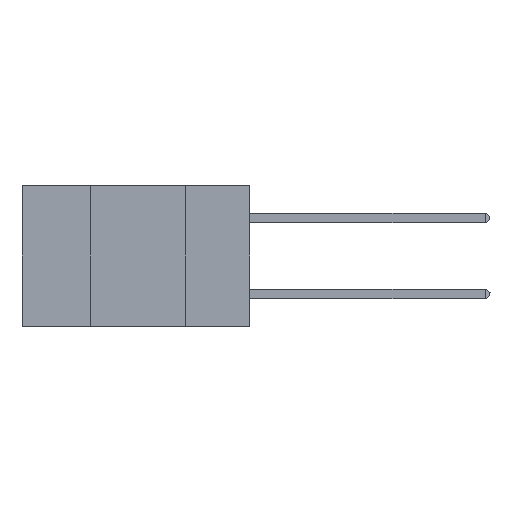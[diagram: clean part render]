
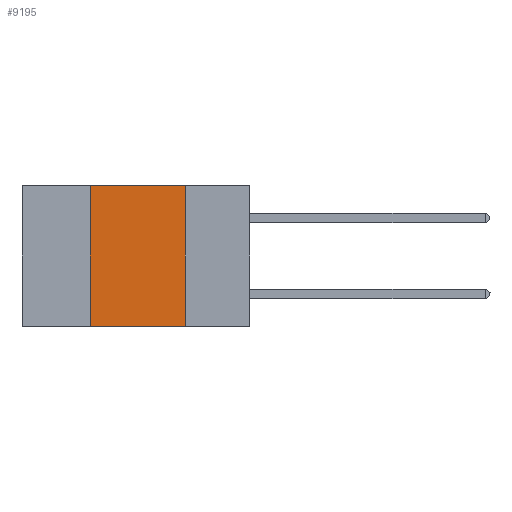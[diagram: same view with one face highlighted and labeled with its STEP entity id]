
A CAD part, left-side view. The second image highlights one B-rep face of the part: STEP entity #9195.
In plain terms, the highlighted planar face has unit normal (-1, 0, 0).
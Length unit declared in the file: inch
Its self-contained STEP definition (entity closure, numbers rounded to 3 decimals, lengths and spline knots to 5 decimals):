
#936 = CARTESIAN_POINT ( 'NONE',  ( 0., 0.6, -0.37 ) ) ;
#1093 = LINE ( 'NONE', #936, #21614 ) ;
#1607 = DIRECTION ( 'NONE',  ( 0., -1., 0. ) ) ;
#2502 = LINE ( 'NONE', #6776, #12777 ) ;
#3246 = CARTESIAN_POINT ( 'NONE',  ( 0., 0.42, 0. ) ) ;
#4138 = VECTOR ( 'NONE', #28139, 39.37008 ) ;
#4332 = ORIENTED_EDGE ( 'NONE', *, *, #9569, .T. ) ;
#4710 = DIRECTION ( 'NONE',  ( 0., 0., -1. ) ) ;
#5427 = DIRECTION ( 'NONE',  ( 0., 0., -1. ) ) ;
#5874 = CARTESIAN_POINT ( 'NONE',  ( 0., 0.42, -0.37 ) ) ;
#6187 = CARTESIAN_POINT ( 'NONE',  ( 0., 0.6, 0. ) ) ;
#6487 = CARTESIAN_POINT ( 'NONE',  ( 0., 0.6, 0. ) ) ;
#6776 = CARTESIAN_POINT ( 'NONE',  ( 0., 0.17, 0. ) ) ;
#7174 = VERTEX_POINT ( 'NONE', #7613 ) ;
#7613 = CARTESIAN_POINT ( 'NONE',  ( 0., 0.42, 0. ) ) ;
#7790 = PLANE ( 'NONE',  #30099 ) ;
#8316 = VERTEX_POINT ( 'NONE', #13761 ) ;
#8860 = VERTEX_POINT ( 'NONE', #16221 ) ;
#9195 = ADVANCED_FACE ( 'NONE', ( #13388 ), #7790, .F. ) ;
#9569 = EDGE_CURVE ( 'NONE', #30423, #8860, #1093, .T. ) ;
#11562 = EDGE_CURVE ( 'NONE', #30423, #7174, #17833, .T. ) ;
#12315 = ORIENTED_EDGE ( 'NONE', *, *, #11562, .F. ) ;
#12777 = VECTOR ( 'NONE', #4710, 39.37008 ) ;
#13388 = FACE_OUTER_BOUND ( 'NONE', #24349, .T. ) ;
#13509 = EDGE_CURVE ( 'NONE', #7174, #8316, #27596, .T. ) ;
#13697 = DIRECTION ( 'NONE',  ( 1., 0., 0. ) ) ;
#13761 = CARTESIAN_POINT ( 'NONE',  ( 0., 0.17, 0. ) ) ;
#15606 = EDGE_CURVE ( 'NONE', #8316, #8860, #2502, .T. ) ;
#16221 = CARTESIAN_POINT ( 'NONE',  ( 0., 0.17, -0.37 ) ) ;
#17833 = LINE ( 'NONE', #3246, #4138 ) ;
#18860 = ORIENTED_EDGE ( 'NONE', *, *, #15606, .F. ) ;
#21614 = VECTOR ( 'NONE', #27864, 39.37008 ) ;
#24349 = EDGE_LOOP ( 'NONE', ( #18860, #28890, #12315, #4332 ) ) ;
#27596 = LINE ( 'NONE', #6187, #28241 ) ;
#27864 = DIRECTION ( 'NONE',  ( 0., -1., 0. ) ) ;
#28139 = DIRECTION ( 'NONE',  ( 0., 0., 1. ) ) ;
#28241 = VECTOR ( 'NONE', #1607, 39.37008 ) ;
#28890 = ORIENTED_EDGE ( 'NONE', *, *, #13509, .F. ) ;
#30099 = AXIS2_PLACEMENT_3D ( 'NONE', #6487, #13697, #5427 ) ;
#30423 = VERTEX_POINT ( 'NONE', #5874 ) ;
